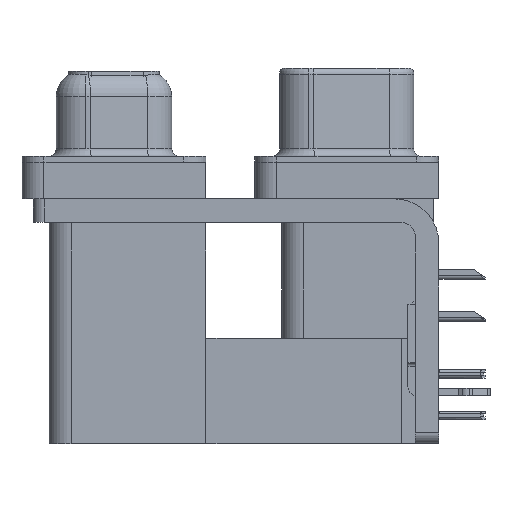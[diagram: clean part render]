
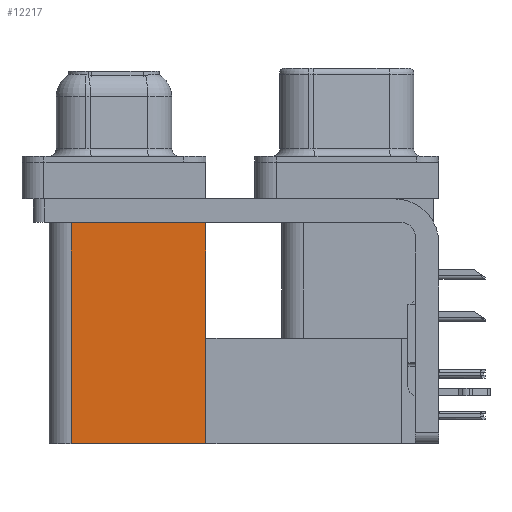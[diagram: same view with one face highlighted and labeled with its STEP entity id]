
A CAD part, left-side view. The second image highlights one B-rep face of the part: STEP entity #12217.
In plain terms, the highlighted planar face has unit normal (-1, 0, 0).
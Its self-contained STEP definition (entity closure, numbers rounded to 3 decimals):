
#2025 = LINE ( 'NONE', #19641, #11913 ) ;
#2231 = EDGE_CURVE ( 'NONE', #31246, #31035, #28978, .T. ) ;
#2942 = VECTOR ( 'NONE', #32182, 1000. ) ;
#4907 = CARTESIAN_POINT ( 'NONE',  ( 3.765, 9.6, -19.2 ) ) ;
#5362 = VERTEX_POINT ( 'NONE', #32718 ) ;
#5758 = EDGE_CURVE ( 'NONE', #5362, #31246, #36368, .T. ) ;
#6781 = DIRECTION ( 'NONE',  ( 0., 1., 0. ) ) ;
#9551 = EDGE_LOOP ( 'NONE', ( #35965, #28361, #15407, #12226 ) ) ;
#9727 = VECTOR ( 'NONE', #25041, 1000. ) ;
#11801 = DIRECTION ( 'NONE',  ( 0., 0., 1. ) ) ;
#11913 = VECTOR ( 'NONE', #11801, 1000. ) ;
#12217 = ADVANCED_FACE ( 'NONE', ( #23205 ), #22515, .F. ) ;
#12226 = ORIENTED_EDGE ( 'NONE', *, *, #17506, .T. ) ;
#15244 = CARTESIAN_POINT ( 'NONE',  ( 3.765, 9.6, -19.2 ) ) ;
#15296 = CARTESIAN_POINT ( 'NONE',  ( 3.765, 9.6, -2.5 ) ) ;
#15407 = ORIENTED_EDGE ( 'NONE', *, *, #5758, .F. ) ;
#16416 = AXIS2_PLACEMENT_3D ( 'NONE', #4907, #22980, #19709 ) ;
#17506 = EDGE_CURVE ( 'NONE', #5362, #21316, #2025, .T. ) ;
#19641 = CARTESIAN_POINT ( 'NONE',  ( 3.765, 9.6, -19.2 ) ) ;
#19709 = DIRECTION ( 'NONE',  ( 0., 0., -1. ) ) ;
#21316 = VERTEX_POINT ( 'NONE', #15296 ) ;
#22515 = PLANE ( 'NONE',  #16416 ) ;
#22980 = DIRECTION ( 'NONE',  ( 1., 0., 0. ) ) ;
#23205 = FACE_OUTER_BOUND ( 'NONE', #9551, .T. ) ;
#24536 = CARTESIAN_POINT ( 'NONE',  ( 3.765, 18.8, -2.5 ) ) ;
#25041 = DIRECTION ( 'NONE',  ( 0., 0., 1. ) ) ;
#27850 = CARTESIAN_POINT ( 'NONE',  ( 3.765, 9.6, -2.5 ) ) ;
#28087 = LINE ( 'NONE', #27850, #42739 ) ;
#28361 = ORIENTED_EDGE ( 'NONE', *, *, #2231, .F. ) ;
#28978 = LINE ( 'NONE', #36185, #9727 ) ;
#31035 = VERTEX_POINT ( 'NONE', #24536 ) ;
#31246 = VERTEX_POINT ( 'NONE', #40785 ) ;
#32182 = DIRECTION ( 'NONE',  ( 0., 1., 0. ) ) ;
#32718 = CARTESIAN_POINT ( 'NONE',  ( 3.765, 9.6, -19.2 ) ) ;
#35965 = ORIENTED_EDGE ( 'NONE', *, *, #43976, .T. ) ;
#36185 = CARTESIAN_POINT ( 'NONE',  ( 3.765, 18.8, -19.2 ) ) ;
#36368 = LINE ( 'NONE', #15244, #2942 ) ;
#40785 = CARTESIAN_POINT ( 'NONE',  ( 3.765, 18.8, -19.2 ) ) ;
#42739 = VECTOR ( 'NONE', #6781, 1000. ) ;
#43976 = EDGE_CURVE ( 'NONE', #21316, #31035, #28087, .T. ) ;
